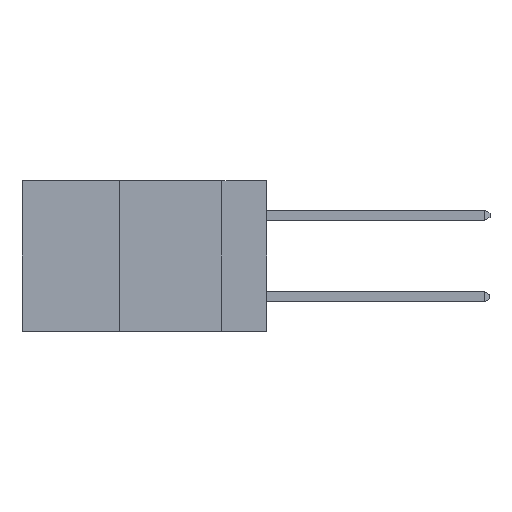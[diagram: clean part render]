
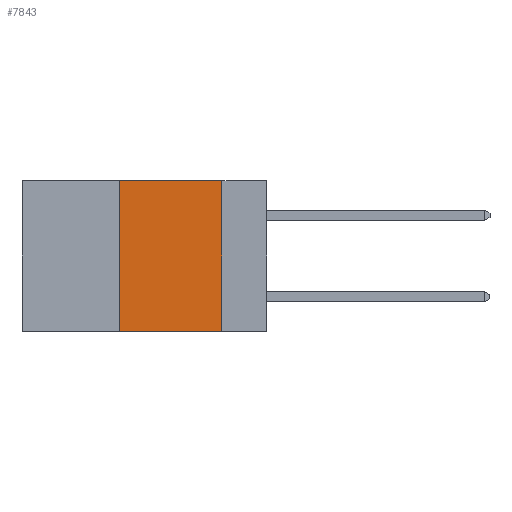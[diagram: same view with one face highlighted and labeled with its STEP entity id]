
A CAD part, left-side view. The second image highlights one B-rep face of the part: STEP entity #7843.
In plain terms, the highlighted planar face has unit normal (-1, 0, 0).
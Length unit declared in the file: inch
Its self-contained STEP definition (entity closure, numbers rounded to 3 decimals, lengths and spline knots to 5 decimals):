
#148 = EDGE_CURVE ( 'NONE', #2134, #6483, #1711, .T. ) ;
#401 = DIRECTION ( 'NONE',  ( 0., 0., 1. ) ) ;
#496 = CARTESIAN_POINT ( 'NONE',  ( 0., 0.36, 0. ) ) ;
#1208 = EDGE_CURVE ( 'NONE', #6483, #7159, #12539, .T. ) ;
#1360 = VECTOR ( 'NONE', #401, 39.37008 ) ;
#1551 = AXIS2_PLACEMENT_3D ( 'NONE', #4904, #13232, #6336 ) ;
#1711 = LINE ( 'NONE', #496, #1360 ) ;
#2054 = CARTESIAN_POINT ( 'NONE',  ( 0., 0.6, 0. ) ) ;
#2134 = VERTEX_POINT ( 'NONE', #8058 ) ;
#2296 = CARTESIAN_POINT ( 'NONE',  ( 0., 0.11, 0. ) ) ;
#2741 = ORIENTED_EDGE ( 'NONE', *, *, #1208, .F. ) ;
#4041 = CARTESIAN_POINT ( 'NONE',  ( 0., 0.6, -0.37 ) ) ;
#4904 = CARTESIAN_POINT ( 'NONE',  ( 0., 0.6, 0. ) ) ;
#5146 = ORIENTED_EDGE ( 'NONE', *, *, #8913, .F. ) ;
#5388 = VECTOR ( 'NONE', #12076, 39.37008 ) ;
#5554 = LINE ( 'NONE', #4041, #5388 ) ;
#6336 = DIRECTION ( 'NONE',  ( 0., 0., -1. ) ) ;
#6483 = VERTEX_POINT ( 'NONE', #9669 ) ;
#7159 = VERTEX_POINT ( 'NONE', #2296 ) ;
#7253 = ORIENTED_EDGE ( 'NONE', *, *, #148, .F. ) ;
#7843 = ADVANCED_FACE ( 'NONE', ( #11848 ), #13077, .F. ) ;
#8058 = CARTESIAN_POINT ( 'NONE',  ( 0., 0.36, -0.37 ) ) ;
#8174 = CARTESIAN_POINT ( 'NONE',  ( 0., 0.11, -0.37 ) ) ;
#8913 = EDGE_CURVE ( 'NONE', #7159, #10054, #14690, .T. ) ;
#9379 = CARTESIAN_POINT ( 'NONE',  ( 0., 0.11, 0. ) ) ;
#9669 = CARTESIAN_POINT ( 'NONE',  ( 0., 0.36, 0. ) ) ;
#10054 = VERTEX_POINT ( 'NONE', #8174 ) ;
#11848 = FACE_OUTER_BOUND ( 'NONE', #13715, .T. ) ;
#12076 = DIRECTION ( 'NONE',  ( 0., -1., 0. ) ) ;
#12212 = DIRECTION ( 'NONE',  ( 0., -1., 0. ) ) ;
#12539 = LINE ( 'NONE', #2054, #14521 ) ;
#12887 = VECTOR ( 'NONE', #13983, 39.37008 ) ;
#13077 = PLANE ( 'NONE',  #1551 ) ;
#13096 = EDGE_CURVE ( 'NONE', #2134, #10054, #5554, .T. ) ;
#13232 = DIRECTION ( 'NONE',  ( 1., 0., 0. ) ) ;
#13715 = EDGE_LOOP ( 'NONE', ( #5146, #2741, #7253, #14575 ) ) ;
#13983 = DIRECTION ( 'NONE',  ( 0., 0., -1. ) ) ;
#14521 = VECTOR ( 'NONE', #12212, 39.37008 ) ;
#14575 = ORIENTED_EDGE ( 'NONE', *, *, #13096, .T. ) ;
#14690 = LINE ( 'NONE', #9379, #12887 ) ;
